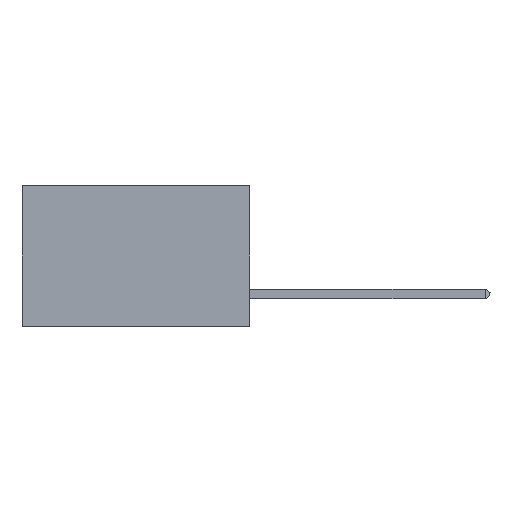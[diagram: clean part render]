
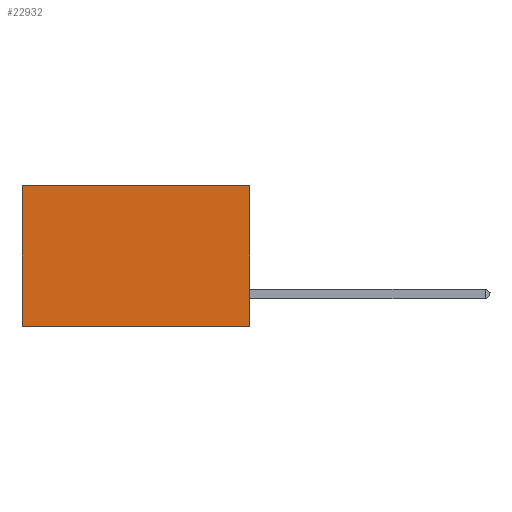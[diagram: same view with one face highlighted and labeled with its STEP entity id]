
A CAD part, left-side view. The second image highlights one B-rep face of the part: STEP entity #22932.
In plain terms, the highlighted planar face has unit normal (-1, 0, 0).
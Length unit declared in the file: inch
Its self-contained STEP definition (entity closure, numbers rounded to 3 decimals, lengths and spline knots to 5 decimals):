
#294 = VERTEX_POINT ( 'NONE', #18517 ) ;
#449 = EDGE_CURVE ( 'NONE', #15818, #17070, #7663, .T. ) ;
#1389 = ORIENTED_EDGE ( 'NONE', *, *, #14394, .T. ) ;
#2056 = ORIENTED_EDGE ( 'NONE', *, *, #19306, .F. ) ;
#2129 = CARTESIAN_POINT ( 'NONE',  ( 0.2875, 0., 0. ) ) ;
#3375 = VECTOR ( 'NONE', #19288, 39.37008 ) ;
#3808 = VECTOR ( 'NONE', #23148, 39.37008 ) ;
#6119 = LINE ( 'NONE', #15340, #3808 ) ;
#7078 = CARTESIAN_POINT ( 'NONE',  ( 0.2875, 0., -0.37 ) ) ;
#7663 = LINE ( 'NONE', #17415, #3375 ) ;
#8741 = VECTOR ( 'NONE', #20020, 39.37008 ) ;
#9399 = ORIENTED_EDGE ( 'NONE', *, *, #23499, .F. ) ;
#9468 = CARTESIAN_POINT ( 'NONE',  ( 0.2875, 0.6, 0. ) ) ;
#9880 = DIRECTION ( 'NONE',  ( 0., 0., -1. ) ) ;
#9990 = DIRECTION ( 'NONE',  ( 0., 0., -1. ) ) ;
#10758 = CARTESIAN_POINT ( 'NONE',  ( 0.2875, 0., 0. ) ) ;
#10798 = LINE ( 'NONE', #7078, #8741 ) ;
#12105 = DIRECTION ( 'NONE',  ( 1., 0., 0. ) ) ;
#14394 = EDGE_CURVE ( 'NONE', #17748, #15818, #6119, .T. ) ;
#14398 = CARTESIAN_POINT ( 'NONE',  ( 0.2875, 0.6, -0.37 ) ) ;
#15340 = CARTESIAN_POINT ( 'NONE',  ( 0.2875, 0., 0. ) ) ;
#15818 = VERTEX_POINT ( 'NONE', #9468 ) ;
#17070 = VERTEX_POINT ( 'NONE', #14398 ) ;
#17415 = CARTESIAN_POINT ( 'NONE',  ( 0.2875, 0.6, 0. ) ) ;
#17432 = CARTESIAN_POINT ( 'NONE',  ( 0.2875, 0., 0. ) ) ;
#17748 = VERTEX_POINT ( 'NONE', #10758 ) ;
#18033 = EDGE_LOOP ( 'NONE', ( #18793, #2056, #9399, #1389 ) ) ;
#18169 = VECTOR ( 'NONE', #9880, 39.37008 ) ;
#18517 = CARTESIAN_POINT ( 'NONE',  ( 0.2875, 0., -0.37 ) ) ;
#18793 = ORIENTED_EDGE ( 'NONE', *, *, #449, .T. ) ;
#19288 = DIRECTION ( 'NONE',  ( 0., 0., -1. ) ) ;
#19306 = EDGE_CURVE ( 'NONE', #294, #17070, #10798, .T. ) ;
#20020 = DIRECTION ( 'NONE',  ( 0., 1., 0. ) ) ;
#20819 = PLANE ( 'NONE',  #22867 ) ;
#22867 = AXIS2_PLACEMENT_3D ( 'NONE', #17432, #12105, #9990 ) ;
#22932 = ADVANCED_FACE ( 'NONE', ( #23364 ), #20819, .F. ) ;
#23148 = DIRECTION ( 'NONE',  ( 0., 1., 0. ) ) ;
#23364 = FACE_OUTER_BOUND ( 'NONE', #18033, .T. ) ;
#23499 = EDGE_CURVE ( 'NONE', #17748, #294, #23630, .T. ) ;
#23630 = LINE ( 'NONE', #2129, #18169 ) ;
